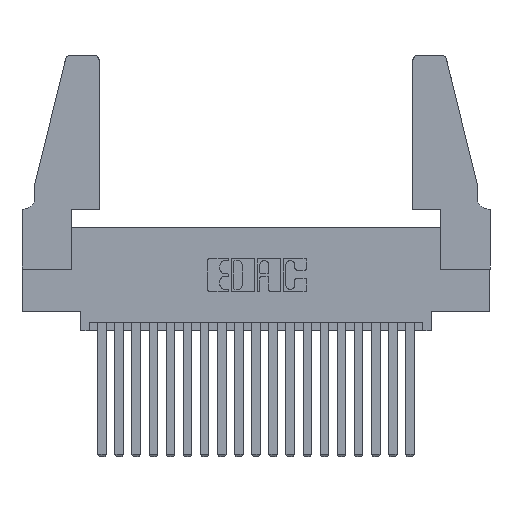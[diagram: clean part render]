
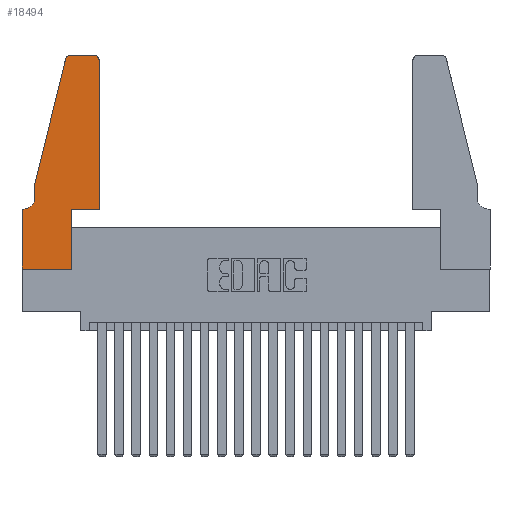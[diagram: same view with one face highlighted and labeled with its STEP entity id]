
A CAD part, top view. The second image highlights one B-rep face of the part: STEP entity #18494.
In plain terms, the highlighted planar face has unit normal (0, 0, 1).
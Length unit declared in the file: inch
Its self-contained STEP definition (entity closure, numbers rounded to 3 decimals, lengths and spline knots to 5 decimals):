
#5 = DIRECTION ( 'NONE',  ( -1., 0., 0. ) ) ;
#285 = DIRECTION ( 'NONE',  ( 0., 0., 1. ) ) ;
#469 = DIRECTION ( 'NONE',  ( 0., -1., 0. ) ) ;
#507 = CARTESIAN_POINT ( 'NONE',  ( 0., 0.35, 0.37 ) ) ;
#892 = CARTESIAN_POINT ( 'NONE',  ( 0., 0., 0.37 ) ) ;
#914 = EDGE_CURVE ( 'NONE', #19394, #6123, #2372, .T. ) ;
#1122 = VECTOR ( 'NONE', #18452, 39.37008 ) ;
#1166 = VERTEX_POINT ( 'NONE', #11466 ) ;
#1330 = CARTESIAN_POINT ( 'NONE',  ( 0.25487, 1.22718, 0.37 ) ) ;
#1474 = CARTESIAN_POINT ( 'NONE',  ( 0.0055, 0.35, 0.37 ) ) ;
#1626 = EDGE_CURVE ( 'NONE', #1166, #17910, #15488, .T. ) ;
#1824 = CIRCLE ( 'NONE', #6087, 0.03 ) ;
#2118 = EDGE_CURVE ( 'NONE', #13042, #7031, #5524, .T. ) ;
#2231 = ORIENTED_EDGE ( 'NONE', *, *, #2118, .T. ) ;
#2239 = CARTESIAN_POINT ( 'NONE',  ( 0.2865, 0.35, 0.37 ) ) ;
#2253 = ORIENTED_EDGE ( 'NONE', *, *, #9001, .T. ) ;
#2372 = LINE ( 'NONE', #17456, #11161 ) ;
#2511 = ORIENTED_EDGE ( 'NONE', *, *, #7570, .T. ) ;
#2577 = CARTESIAN_POINT ( 'NONE',  ( 0.4505, 1.22, 0.37 ) ) ;
#2751 = EDGE_CURVE ( 'NONE', #17910, #19394, #8631, .T. ) ;
#3184 = DIRECTION ( 'NONE',  ( 0., 0., -1. ) ) ;
#3282 = CARTESIAN_POINT ( 'NONE',  ( 0.284, 1.25, 0.37 ) ) ;
#3917 = DIRECTION ( 'NONE',  ( 1., 0., 0. ) ) ;
#3934 = LINE ( 'NONE', #13534, #15119 ) ;
#3972 = EDGE_LOOP ( 'NONE', ( #2511, #2231, #6097, #6397, #5680, #8673, #12075, #6513, #15654, #17754, #13230, #2253 ) ) ;
#4159 = CARTESIAN_POINT ( 'NONE',  ( 0.4505, 0.35, 0.37 ) ) ;
#4461 = DIRECTION ( 'NONE',  ( -1., 0., 0. ) ) ;
#5115 = CARTESIAN_POINT ( 'NONE',  ( 0.4205, 1.25, 0.37 ) ) ;
#5162 = DIRECTION ( 'NONE',  ( 1., 0., 0. ) ) ;
#5402 = LINE ( 'NONE', #4159, #16082 ) ;
#5524 = CIRCLE ( 'NONE', #17211, 0.03 ) ;
#5680 = ORIENTED_EDGE ( 'NONE', *, *, #1626, .T. ) ;
#5811 = DIRECTION ( 'NONE',  ( 0., 1., 0. ) ) ;
#5932 = LINE ( 'NONE', #19161, #16123 ) ;
#6087 = AXIS2_PLACEMENT_3D ( 'NONE', #12410, #12618, #9489 ) ;
#6097 = ORIENTED_EDGE ( 'NONE', *, *, #9235, .T. ) ;
#6123 = VERTEX_POINT ( 'NONE', #892 ) ;
#6165 = LINE ( 'NONE', #16419, #13942 ) ;
#6223 = CARTESIAN_POINT ( 'NONE',  ( 0.0755, 0.35, 0.37 ) ) ;
#6337 = VERTEX_POINT ( 'NONE', #2239 ) ;
#6354 = CARTESIAN_POINT ( 'NONE',  ( 0., 0., 0.37 ) ) ;
#6397 = ORIENTED_EDGE ( 'NONE', *, *, #9958, .T. ) ;
#6513 = ORIENTED_EDGE ( 'NONE', *, *, #19334, .T. ) ;
#6970 = CARTESIAN_POINT ( 'NONE',  ( 0.0755, 0.5, 0.37 ) ) ;
#7031 = VERTEX_POINT ( 'NONE', #1330 ) ;
#7196 = DIRECTION ( 'NONE',  ( 0., 1., 0. ) ) ;
#7570 = EDGE_CURVE ( 'NONE', #10077, #13042, #8362, .T. ) ;
#8116 = VERTEX_POINT ( 'NONE', #2577 ) ;
#8252 = LINE ( 'NONE', #6354, #11944 ) ;
#8362 = LINE ( 'NONE', #10925, #9617 ) ;
#8533 = DIRECTION ( 'NONE',  ( 0., -1., 0. ) ) ;
#8631 = LINE ( 'NONE', #6223, #1122 ) ;
#8673 = ORIENTED_EDGE ( 'NONE', *, *, #2751, .T. ) ;
#9001 = EDGE_CURVE ( 'NONE', #8116, #10077, #1824, .T. ) ;
#9136 = VERTEX_POINT ( 'NONE', #15462 ) ;
#9235 = EDGE_CURVE ( 'NONE', #7031, #13708, #6165, .T. ) ;
#9315 = CARTESIAN_POINT ( 'NONE',  ( 0.0055, 0.42, 0.37 ) ) ;
#9489 = DIRECTION ( 'NONE',  ( 1., 0., 0. ) ) ;
#9617 = VECTOR ( 'NONE', #4461, 39.37008 ) ;
#9958 = EDGE_CURVE ( 'NONE', #13708, #1166, #19026, .T. ) ;
#10077 = VERTEX_POINT ( 'NONE', #5115 ) ;
#10339 = EDGE_CURVE ( 'NONE', #19132, #6337, #5932, .T. ) ;
#10445 = DIRECTION ( 'NONE',  ( -0.239, -0.971, 0. ) ) ;
#10925 = CARTESIAN_POINT ( 'NONE',  ( 0.2605, 1.25, 0.37 ) ) ;
#11010 = VECTOR ( 'NONE', #8533, 39.37008 ) ;
#11161 = VECTOR ( 'NONE', #469, 39.37008 ) ;
#11466 = CARTESIAN_POINT ( 'NONE',  ( 0.0755, 0.42, 0.37 ) ) ;
#11607 = AXIS2_PLACEMENT_3D ( 'NONE', #9315, #3184, #5 ) ;
#11944 = VECTOR ( 'NONE', #19127, 39.37008 ) ;
#12028 = EDGE_CURVE ( 'NONE', #9136, #8116, #5402, .T. ) ;
#12071 = EDGE_CURVE ( 'NONE', #6337, #9136, #3934, .T. ) ;
#12075 = ORIENTED_EDGE ( 'NONE', *, *, #914, .T. ) ;
#12410 = CARTESIAN_POINT ( 'NONE',  ( 0.4205, 1.22, 0.37 ) ) ;
#12618 = DIRECTION ( 'NONE',  ( 0., 0., 1. ) ) ;
#12969 = PLANE ( 'NONE',  #16806 ) ;
#13042 = VERTEX_POINT ( 'NONE', #3282 ) ;
#13230 = ORIENTED_EDGE ( 'NONE', *, *, #12028, .T. ) ;
#13534 = CARTESIAN_POINT ( 'NONE',  ( 0.4505, 0.35, 0.37 ) ) ;
#13708 = VERTEX_POINT ( 'NONE', #15699 ) ;
#13942 = VECTOR ( 'NONE', #10445, 39.37008 ) ;
#15119 = VECTOR ( 'NONE', #15220, 39.37008 ) ;
#15220 = DIRECTION ( 'NONE',  ( 1., 0., 0. ) ) ;
#15462 = CARTESIAN_POINT ( 'NONE',  ( 0.4505, 0.35, 0.37 ) ) ;
#15488 = CIRCLE ( 'NONE', #11607, 0.07 ) ;
#15654 = ORIENTED_EDGE ( 'NONE', *, *, #10339, .T. ) ;
#15699 = CARTESIAN_POINT ( 'NONE',  ( 0.0755, 0.5, 0.37 ) ) ;
#15845 = FACE_OUTER_BOUND ( 'NONE', #3972, .T. ) ;
#16082 = VECTOR ( 'NONE', #5811, 39.37008 ) ;
#16123 = VECTOR ( 'NONE', #7196, 39.37008 ) ;
#16419 = CARTESIAN_POINT ( 'NONE',  ( 0.0755, 0.5, 0.37 ) ) ;
#16806 = AXIS2_PLACEMENT_3D ( 'NONE', #19024, #285, #5162 ) ;
#17044 = CARTESIAN_POINT ( 'NONE',  ( 0.2865, 0., 0.37 ) ) ;
#17211 = AXIS2_PLACEMENT_3D ( 'NONE', #17914, #19333, #3917 ) ;
#17456 = CARTESIAN_POINT ( 'NONE',  ( 0., 0., 0.37 ) ) ;
#17754 = ORIENTED_EDGE ( 'NONE', *, *, #12071, .T. ) ;
#17910 = VERTEX_POINT ( 'NONE', #1474 ) ;
#17914 = CARTESIAN_POINT ( 'NONE',  ( 0.284, 1.22, 0.37 ) ) ;
#18452 = DIRECTION ( 'NONE',  ( -1., 0., 0. ) ) ;
#18494 = ADVANCED_FACE ( 'NONE', ( #15845 ), #12969, .T. ) ;
#19024 = CARTESIAN_POINT ( 'NONE',  ( 0., 0.35, 0.37 ) ) ;
#19026 = LINE ( 'NONE', #6970, #11010 ) ;
#19127 = DIRECTION ( 'NONE',  ( 1., 0., 0. ) ) ;
#19132 = VERTEX_POINT ( 'NONE', #17044 ) ;
#19161 = CARTESIAN_POINT ( 'NONE',  ( 0.2865, 0.35, 0.37 ) ) ;
#19333 = DIRECTION ( 'NONE',  ( 0., 0., 1. ) ) ;
#19334 = EDGE_CURVE ( 'NONE', #6123, #19132, #8252, .T. ) ;
#19394 = VERTEX_POINT ( 'NONE', #507 ) ;
